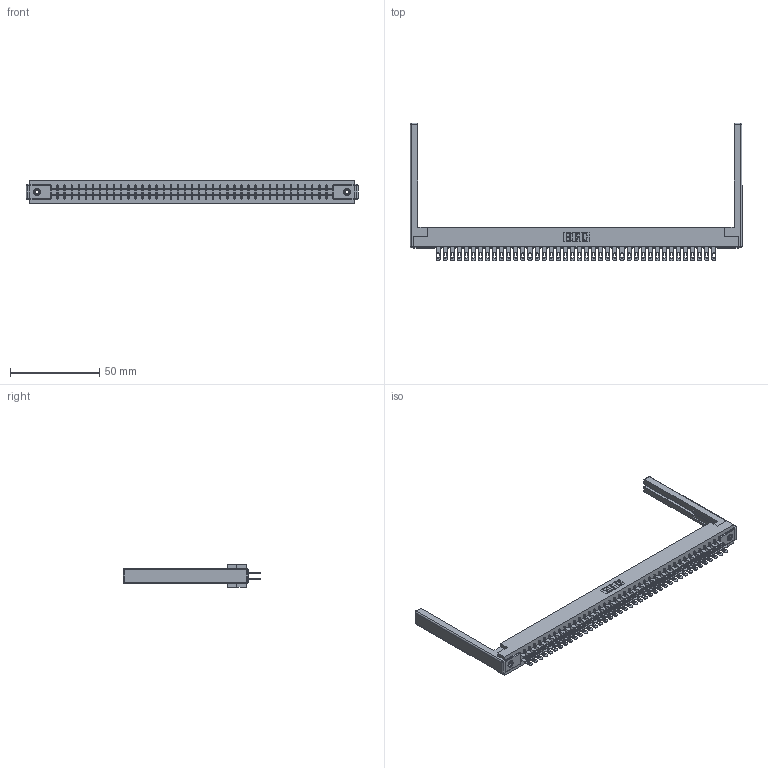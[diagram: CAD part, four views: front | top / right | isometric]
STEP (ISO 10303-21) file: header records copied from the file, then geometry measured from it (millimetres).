
FILE_DESCRIPTION (( 'STEP AP203' ), '1' );
FILE_NAME ('305-080-500-568.STEP', '2019-09-10T09:41:37', ( '' ), ( '' ), 'SwSTEP 2.0', 'SolidWorks 2016', '' );
FILE_SCHEMA (( 'CONFIG_CONTROL_DESIGN' ));
Length unit declared in the file: inch
Products named in the file (5): 305-080-500-568; 305 Part_.156 Dia; 345-250-001_345-250-001-102; 305-290-001_500; 307-220-068
Assembly tree (85 placements, depth 2):
  305-080-500-568
    305 Part_.156 Dia
    305-290-001_500  x80
    345-250-001_345-250-001-102  x2
    307-220-068  x2
Bounding box: 185.93 x 77.14 x 12.7 mm (x, y, z)
Volume: 23468.5 mm3; surface area: 30649.2 mm2
Topology: 85 solids, 85 shells, 4270 faces, 12186 edges, 7888 vertices
Faces by surface type: plane 2396, cylinder 1690, sphere 168, cone 12, torus 4
Entity records: 46334 total; most frequent: CARTESIAN_POINT 7639, ORIENTED_EDGE 7574, DIRECTION 7413, EDGE_CURVE 3787, LINE 3049, VECTOR 3049, VERTEX_POINT 2408, AXIS2_PLACEMENT_3D 2182
